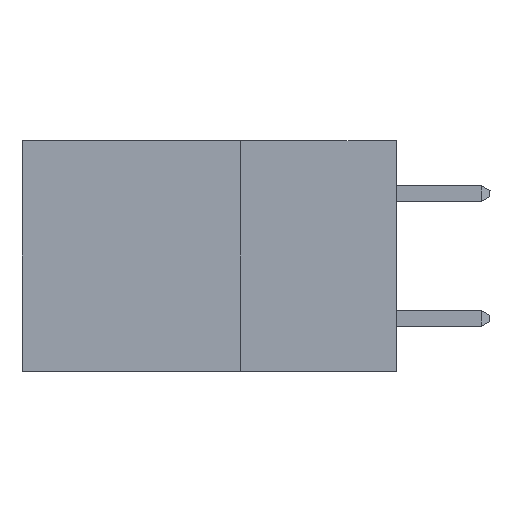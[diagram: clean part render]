
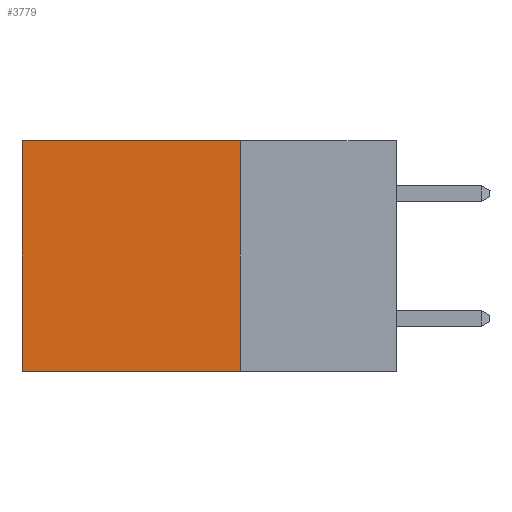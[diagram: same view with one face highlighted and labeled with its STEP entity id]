
A CAD part, left-side view. The second image highlights one B-rep face of the part: STEP entity #3779.
In plain terms, the highlighted planar face has unit normal (-1, 0, 0).
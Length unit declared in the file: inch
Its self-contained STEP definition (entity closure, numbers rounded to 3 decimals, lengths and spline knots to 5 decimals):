
#564 = DIRECTION ( 'NONE',  ( 0., 0., -1. ) ) ;
#631 = CARTESIAN_POINT ( 'NONE',  ( 0.298, 0.25, 0. ) ) ;
#1340 = FACE_OUTER_BOUND ( 'NONE', #3148, .T. ) ;
#2233 = PLANE ( 'NONE',  #13357 ) ;
#2680 = CARTESIAN_POINT ( 'NONE',  ( 0.298, 0.6, -0.37 ) ) ;
#2964 = EDGE_CURVE ( 'NONE', #13192, #9755, #13950, .T. ) ;
#3148 = EDGE_LOOP ( 'NONE', ( #3928, #3170, #15776, #10997 ) ) ;
#3157 = VECTOR ( 'NONE', #13640, 39.37008 ) ;
#3170 = ORIENTED_EDGE ( 'NONE', *, *, #3688, .F. ) ;
#3688 = EDGE_CURVE ( 'NONE', #9755, #9498, #17245, .T. ) ;
#3779 = ADVANCED_FACE ( 'NONE', ( #1340 ), #2233, .F. ) ;
#3928 = ORIENTED_EDGE ( 'NONE', *, *, #17420, .T. ) ;
#7219 = VECTOR ( 'NONE', #17895, 39.37008 ) ;
#9075 = CARTESIAN_POINT ( 'NONE',  ( 0.298, 0.6, 0. ) ) ;
#9498 = VERTEX_POINT ( 'NONE', #2680 ) ;
#9755 = VERTEX_POINT ( 'NONE', #11647 ) ;
#9764 = VECTOR ( 'NONE', #10693, 39.37008 ) ;
#10461 = CARTESIAN_POINT ( 'NONE',  ( 0.298, 0.25, -0.37 ) ) ;
#10693 = DIRECTION ( 'NONE',  ( 0., 1., 0. ) ) ;
#10915 = LINE ( 'NONE', #13592, #7219 ) ;
#10997 = ORIENTED_EDGE ( 'NONE', *, *, #16771, .T. ) ;
#11612 = DIRECTION ( 'NONE',  ( 1., 0., 0. ) ) ;
#11647 = CARTESIAN_POINT ( 'NONE',  ( 0.298, 0.25, -0.37 ) ) ;
#11687 = VERTEX_POINT ( 'NONE', #9075 ) ;
#11971 = CARTESIAN_POINT ( 'NONE',  ( 0.298, 0.25, 0. ) ) ;
#13192 = VERTEX_POINT ( 'NONE', #14279 ) ;
#13357 = AXIS2_PLACEMENT_3D ( 'NONE', #11971, #11612, #17514 ) ;
#13592 = CARTESIAN_POINT ( 'NONE',  ( 0.298, 0.25, 0. ) ) ;
#13640 = DIRECTION ( 'NONE',  ( 0., 0., -1. ) ) ;
#13950 = LINE ( 'NONE', #631, #14413 ) ;
#14279 = CARTESIAN_POINT ( 'NONE',  ( 0.298, 0.25, 0. ) ) ;
#14413 = VECTOR ( 'NONE', #564, 39.37008 ) ;
#15776 = ORIENTED_EDGE ( 'NONE', *, *, #2964, .F. ) ;
#16771 = EDGE_CURVE ( 'NONE', #13192, #11687, #10915, .T. ) ;
#17245 = LINE ( 'NONE', #10461, #9764 ) ;
#17420 = EDGE_CURVE ( 'NONE', #11687, #9498, #18162, .T. ) ;
#17514 = DIRECTION ( 'NONE',  ( 0., 0., -1. ) ) ;
#17816 = CARTESIAN_POINT ( 'NONE',  ( 0.298, 0.6, 0. ) ) ;
#17895 = DIRECTION ( 'NONE',  ( 0., 1., 0. ) ) ;
#18162 = LINE ( 'NONE', #17816, #3157 ) ;
